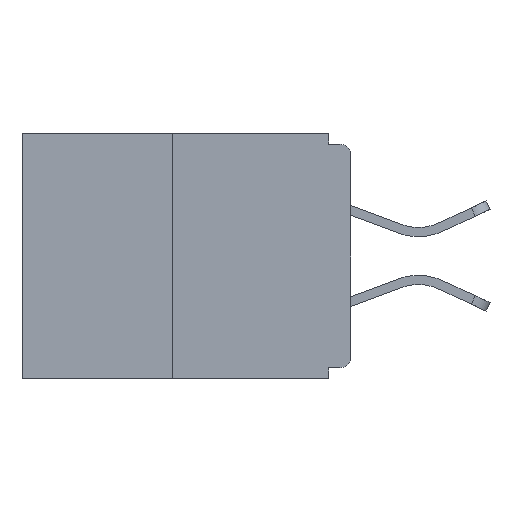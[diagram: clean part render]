
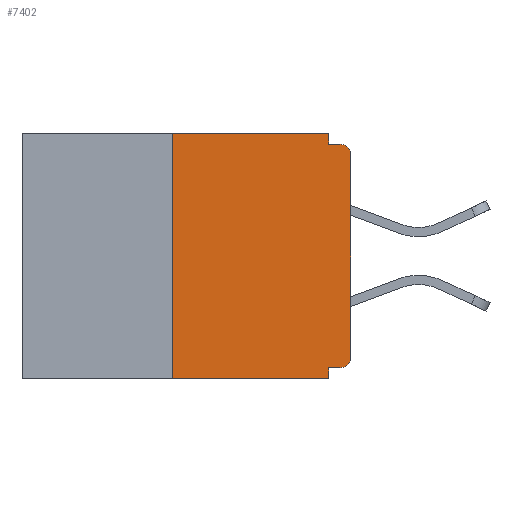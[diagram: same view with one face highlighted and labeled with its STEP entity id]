
A CAD part, left-side view. The second image highlights one B-rep face of the part: STEP entity #7402.
In plain terms, the highlighted planar face has unit normal (-1, 0, 0).
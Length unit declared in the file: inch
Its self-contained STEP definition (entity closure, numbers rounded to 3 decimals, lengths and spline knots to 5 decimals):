
#25 = CARTESIAN_POINT ( 'NONE',  ( 0., 0.46, 0. ) ) ;
#111 = PLANE ( 'NONE',  #11524 ) ;
#148 = VECTOR ( 'NONE', #10812, 39.37008 ) ;
#254 = ORIENTED_EDGE ( 'NONE', *, *, #6113, .F. ) ;
#361 = LINE ( 'NONE', #9381, #10592 ) ;
#734 = LINE ( 'NONE', #4357, #787 ) ;
#787 = VECTOR ( 'NONE', #10655, 39.37008 ) ;
#859 = DIRECTION ( 'NONE',  ( 0., 0., 1. ) ) ;
#896 = EDGE_CURVE ( 'NONE', #12094, #13554, #910, .T. ) ;
#910 = CIRCLE ( 'NONE', #9366, 0.015 ) ;
#1010 = CARTESIAN_POINT ( 'NONE',  ( 0., 0., 0. ) ) ;
#1391 = CARTESIAN_POINT ( 'NONE',  ( 0., 0.031, -0.328 ) ) ;
#1478 = ORIENTED_EDGE ( 'NONE', *, *, #8832, .T. ) ;
#1990 = ORIENTED_EDGE ( 'NONE', *, *, #14565, .F. ) ;
#2343 = LINE ( 'NONE', #12103, #10365 ) ;
#2413 = ORIENTED_EDGE ( 'NONE', *, *, #4316, .F. ) ;
#2417 = VECTOR ( 'NONE', #859, 39.37008 ) ;
#3046 = CARTESIAN_POINT ( 'NONE',  ( 0., 0.015, -0.03 ) ) ;
#3110 = DIRECTION ( 'NONE',  ( 0., -1., 0. ) ) ;
#3426 = VECTOR ( 'NONE', #8504, 39.37008 ) ;
#3543 = CARTESIAN_POINT ( 'NONE',  ( 0., 0.031, -0.343 ) ) ;
#3788 = EDGE_LOOP ( 'NONE', ( #1990, #254, #10582, #2413, #11636, #11034, #1478, #9191, #8256, #7495 ) ) ;
#4316 = EDGE_CURVE ( 'NONE', #14408, #6225, #14868, .T. ) ;
#4357 = CARTESIAN_POINT ( 'NONE',  ( 0., 0., -0.328 ) ) ;
#4980 = EDGE_CURVE ( 'NONE', #9733, #8858, #8565, .T. ) ;
#5015 = VERTEX_POINT ( 'NONE', #10767 ) ;
#5137 = DIRECTION ( 'NONE',  ( 1., 0., 0. ) ) ;
#5990 = EDGE_CURVE ( 'NONE', #5015, #6225, #361, .T. ) ;
#6113 = EDGE_CURVE ( 'NONE', #5015, #10557, #10697, .T. ) ;
#6172 = AXIS2_PLACEMENT_3D ( 'NONE', #15661, #9617, #12084 ) ;
#6225 = VERTEX_POINT ( 'NONE', #13958 ) ;
#6238 = CARTESIAN_POINT ( 'NONE',  ( 0., 0., -0.015 ) ) ;
#6913 = VERTEX_POINT ( 'NONE', #16089 ) ;
#7402 = ADVANCED_FACE ( 'NONE', ( #11436 ), #111, .F. ) ;
#7495 = ORIENTED_EDGE ( 'NONE', *, *, #12475, .F. ) ;
#7924 = DIRECTION ( 'NONE',  ( -1., 0., 0. ) ) ;
#8256 = ORIENTED_EDGE ( 'NONE', *, *, #14191, .F. ) ;
#8504 = DIRECTION ( 'NONE',  ( 0., -1., 0. ) ) ;
#8560 = EDGE_CURVE ( 'NONE', #9733, #14408, #734, .T. ) ;
#8565 = CIRCLE ( 'NONE', #6172, 0.015 ) ;
#8715 = CARTESIAN_POINT ( 'NONE',  ( 0., 0., -0.03 ) ) ;
#8832 = EDGE_CURVE ( 'NONE', #8858, #12094, #12179, .T. ) ;
#8858 = VERTEX_POINT ( 'NONE', #9709 ) ;
#9191 = ORIENTED_EDGE ( 'NONE', *, *, #896, .T. ) ;
#9209 = DIRECTION ( 'NONE',  ( 0., -1., 0. ) ) ;
#9366 = AXIS2_PLACEMENT_3D ( 'NONE', #3046, #7924, #13136 ) ;
#9381 = CARTESIAN_POINT ( 'NONE',  ( 0., 0.46, -0.343 ) ) ;
#9388 = CARTESIAN_POINT ( 'NONE',  ( 0., 0.25, 0. ) ) ;
#9410 = LINE ( 'NONE', #12039, #14258 ) ;
#9617 = DIRECTION ( 'NONE',  ( -1., 0., 0. ) ) ;
#9709 = CARTESIAN_POINT ( 'NONE',  ( 0., 0., -0.313 ) ) ;
#9733 = VERTEX_POINT ( 'NONE', #14725 ) ;
#9881 = DIRECTION ( 'NONE',  ( 0., 0., -1. ) ) ;
#10365 = VECTOR ( 'NONE', #9881, 39.37008 ) ;
#10557 = VERTEX_POINT ( 'NONE', #9388 ) ;
#10582 = ORIENTED_EDGE ( 'NONE', *, *, #5990, .T. ) ;
#10592 = VECTOR ( 'NONE', #9209, 39.37008 ) ;
#10655 = DIRECTION ( 'NONE',  ( 0., 1., 0. ) ) ;
#10697 = LINE ( 'NONE', #15819, #2417 ) ;
#10767 = CARTESIAN_POINT ( 'NONE',  ( 0., 0.25, -0.343 ) ) ;
#10812 = DIRECTION ( 'NONE',  ( 0., 0., -1. ) ) ;
#11034 = ORIENTED_EDGE ( 'NONE', *, *, #4980, .T. ) ;
#11436 = FACE_OUTER_BOUND ( 'NONE', #3788, .T. ) ;
#11524 = AXIS2_PLACEMENT_3D ( 'NONE', #25, #5137, #15082 ) ;
#11636 = ORIENTED_EDGE ( 'NONE', *, *, #8560, .F. ) ;
#11660 = CARTESIAN_POINT ( 'NONE',  ( 0., 0.031, 0. ) ) ;
#12039 = CARTESIAN_POINT ( 'NONE',  ( 0., 0.46, 0. ) ) ;
#12084 = DIRECTION ( 'NONE',  ( 0., 0., -1. ) ) ;
#12094 = VERTEX_POINT ( 'NONE', #8715 ) ;
#12103 = CARTESIAN_POINT ( 'NONE',  ( 0., 0.031, 0. ) ) ;
#12179 = LINE ( 'NONE', #1010, #13216 ) ;
#12315 = LINE ( 'NONE', #6238, #3426 ) ;
#12423 = CARTESIAN_POINT ( 'NONE',  ( 0., 0.015, -0.015 ) ) ;
#12475 = EDGE_CURVE ( 'NONE', #15306, #6913, #2343, .T. ) ;
#13136 = DIRECTION ( 'NONE',  ( 0., 0., -1. ) ) ;
#13216 = VECTOR ( 'NONE', #15996, 39.37008 ) ;
#13554 = VERTEX_POINT ( 'NONE', #12423 ) ;
#13958 = CARTESIAN_POINT ( 'NONE',  ( 0., 0.031, -0.343 ) ) ;
#14191 = EDGE_CURVE ( 'NONE', #6913, #13554, #12315, .T. ) ;
#14258 = VECTOR ( 'NONE', #3110, 39.37008 ) ;
#14408 = VERTEX_POINT ( 'NONE', #1391 ) ;
#14565 = EDGE_CURVE ( 'NONE', #10557, #15306, #9410, .T. ) ;
#14725 = CARTESIAN_POINT ( 'NONE',  ( 0., 0.015, -0.328 ) ) ;
#14868 = LINE ( 'NONE', #3543, #148 ) ;
#15082 = DIRECTION ( 'NONE',  ( 0., 0., -1. ) ) ;
#15306 = VERTEX_POINT ( 'NONE', #11660 ) ;
#15661 = CARTESIAN_POINT ( 'NONE',  ( 0., 0.015, -0.313 ) ) ;
#15819 = CARTESIAN_POINT ( 'NONE',  ( 0., 0.25, 0. ) ) ;
#15996 = DIRECTION ( 'NONE',  ( 0., 0., 1. ) ) ;
#16089 = CARTESIAN_POINT ( 'NONE',  ( 0., 0.031, -0.015 ) ) ;
